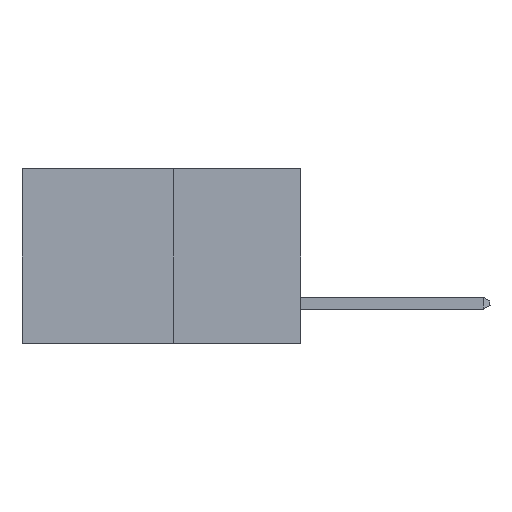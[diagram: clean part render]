
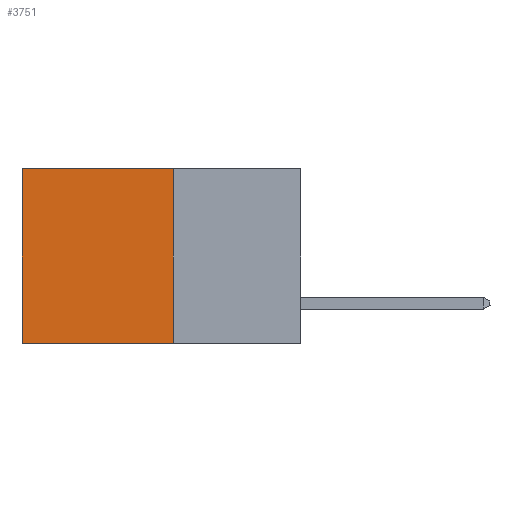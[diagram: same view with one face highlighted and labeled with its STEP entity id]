
A CAD part, left-side view. The second image highlights one B-rep face of the part: STEP entity #3751.
In plain terms, the highlighted planar face has unit normal (-1, 0, 0).
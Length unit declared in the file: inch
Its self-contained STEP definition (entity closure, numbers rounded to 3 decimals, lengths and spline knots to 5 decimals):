
#209 = LINE ( 'NONE', #10746, #2491 ) ;
#252 = EDGE_LOOP ( 'NONE', ( #6705, #5169, #4652, #5505 ) ) ;
#330 = CARTESIAN_POINT ( 'NONE',  ( 0.277, 0.59, -0.37 ) ) ;
#1101 = LINE ( 'NONE', #8267, #8488 ) ;
#1262 = VERTEX_POINT ( 'NONE', #330 ) ;
#1317 = CARTESIAN_POINT ( 'NONE',  ( 0.277, 0.59, 0. ) ) ;
#2008 = CARTESIAN_POINT ( 'NONE',  ( 0.277, 0.27, -0.37 ) ) ;
#2232 = DIRECTION ( 'NONE',  ( 0., 0., -1. ) ) ;
#2342 = LINE ( 'NONE', #9952, #4346 ) ;
#2437 = VECTOR ( 'NONE', #6420, 39.37008 ) ;
#2491 = VECTOR ( 'NONE', #2232, 39.37008 ) ;
#2514 = DIRECTION ( 'NONE',  ( 0., 0., -1. ) ) ;
#3271 = CARTESIAN_POINT ( 'NONE',  ( 0.277, 0.27, 0. ) ) ;
#3751 = ADVANCED_FACE ( 'NONE', ( #7680 ), #5859, .F. ) ;
#4227 = CARTESIAN_POINT ( 'NONE',  ( 0.277, 0.27, 0. ) ) ;
#4346 = VECTOR ( 'NONE', #10885, 39.37008 ) ;
#4652 = ORIENTED_EDGE ( 'NONE', *, *, #5100, .F. ) ;
#4836 = DIRECTION ( 'NONE',  ( 1., 0., 0. ) ) ;
#5083 = LINE ( 'NONE', #4227, #2437 ) ;
#5100 = EDGE_CURVE ( 'NONE', #7422, #7197, #209, .T. ) ;
#5169 = ORIENTED_EDGE ( 'NONE', *, *, #7973, .F. ) ;
#5369 = EDGE_CURVE ( 'NONE', #11225, #1262, #2342, .T. ) ;
#5505 = ORIENTED_EDGE ( 'NONE', *, *, #9546, .T. ) ;
#5775 = CARTESIAN_POINT ( 'NONE',  ( 0.277, 0.27, -0.37 ) ) ;
#5859 = PLANE ( 'NONE',  #10773 ) ;
#6420 = DIRECTION ( 'NONE',  ( 0., 1., 0. ) ) ;
#6705 = ORIENTED_EDGE ( 'NONE', *, *, #5369, .T. ) ;
#7197 = VERTEX_POINT ( 'NONE', #5775 ) ;
#7422 = VERTEX_POINT ( 'NONE', #3271 ) ;
#7680 = FACE_OUTER_BOUND ( 'NONE', #252, .T. ) ;
#7973 = EDGE_CURVE ( 'NONE', #7197, #1262, #1101, .T. ) ;
#8214 = DIRECTION ( 'NONE',  ( 0., 1., 0. ) ) ;
#8267 = CARTESIAN_POINT ( 'NONE',  ( 0.277, 0.27, -0.37 ) ) ;
#8488 = VECTOR ( 'NONE', #8214, 39.37008 ) ;
#9546 = EDGE_CURVE ( 'NONE', #7422, #11225, #5083, .T. ) ;
#9952 = CARTESIAN_POINT ( 'NONE',  ( 0.277, 0.59, -0.37 ) ) ;
#10746 = CARTESIAN_POINT ( 'NONE',  ( 0.277, 0.27, -0.37 ) ) ;
#10773 = AXIS2_PLACEMENT_3D ( 'NONE', #2008, #4836, #2514 ) ;
#10885 = DIRECTION ( 'NONE',  ( 0., 0., -1. ) ) ;
#11225 = VERTEX_POINT ( 'NONE', #1317 ) ;
